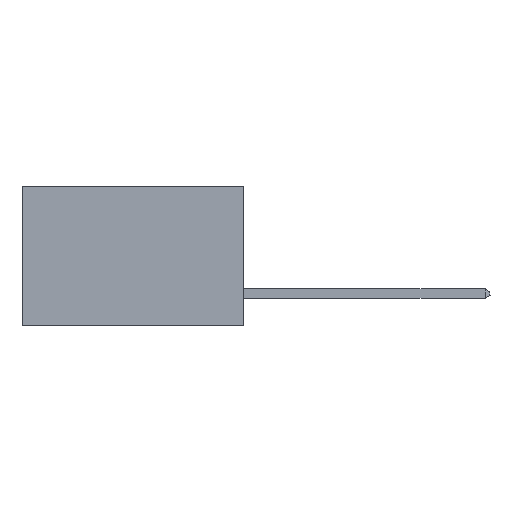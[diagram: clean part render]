
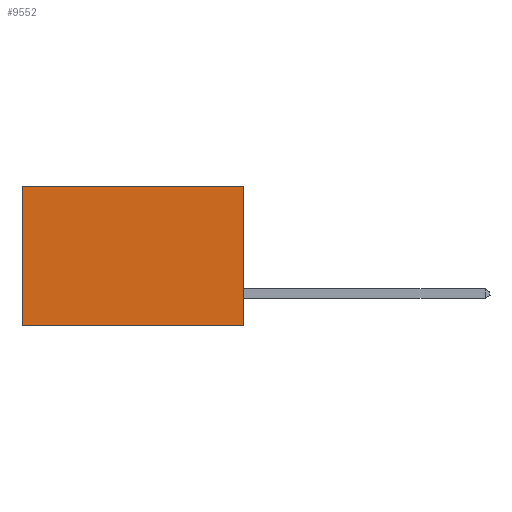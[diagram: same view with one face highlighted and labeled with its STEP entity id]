
A CAD part, left-side view. The second image highlights one B-rep face of the part: STEP entity #9552.
In plain terms, the highlighted planar face has unit normal (-1, 0, 0).
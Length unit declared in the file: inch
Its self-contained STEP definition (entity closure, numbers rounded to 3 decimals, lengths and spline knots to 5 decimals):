
#828 = CARTESIAN_POINT ( 'NONE',  ( 0.277, 0.59, 0. ) ) ;
#1208 = LINE ( 'NONE', #3026, #3178 ) ;
#1336 = EDGE_CURVE ( 'NONE', #2135, #3964, #9751, .T. ) ;
#1589 = LINE ( 'NONE', #7662, #7437 ) ;
#1812 = CARTESIAN_POINT ( 'NONE',  ( 0.277, 0., 0. ) ) ;
#2074 = VERTEX_POINT ( 'NONE', #828 ) ;
#2135 = VERTEX_POINT ( 'NONE', #4495 ) ;
#2694 = CARTESIAN_POINT ( 'NONE',  ( 0.277, 0., -0.37 ) ) ;
#3010 = DIRECTION ( 'NONE',  ( 0., 0., -1. ) ) ;
#3026 = CARTESIAN_POINT ( 'NONE',  ( 0.277, 0.59, -0.37 ) ) ;
#3117 = FACE_OUTER_BOUND ( 'NONE', #6435, .T. ) ;
#3178 = VECTOR ( 'NONE', #3010, 39.37008 ) ;
#3226 = EDGE_CURVE ( 'NONE', #4968, #2074, #1589, .T. ) ;
#3503 = VECTOR ( 'NONE', #6865, 39.37008 ) ;
#3539 = DIRECTION ( 'NONE',  ( 1., 0., 0. ) ) ;
#3964 = VERTEX_POINT ( 'NONE', #8629 ) ;
#4495 = CARTESIAN_POINT ( 'NONE',  ( 0.277, 0., -0.37 ) ) ;
#4794 = EDGE_CURVE ( 'NONE', #2074, #3964, #1208, .T. ) ;
#4968 = VERTEX_POINT ( 'NONE', #1812 ) ;
#5439 = DIRECTION ( 'NONE',  ( 0., 1., 0. ) ) ;
#5624 = ORIENTED_EDGE ( 'NONE', *, *, #1336, .F. ) ;
#5736 = AXIS2_PLACEMENT_3D ( 'NONE', #2694, #3539, #8880 ) ;
#5747 = CARTESIAN_POINT ( 'NONE',  ( 0.277, 0., -0.37 ) ) ;
#6435 = EDGE_LOOP ( 'NONE', ( #9334, #5624, #7628, #9555 ) ) ;
#6865 = DIRECTION ( 'NONE',  ( 0., 0., -1. ) ) ;
#7428 = PLANE ( 'NONE',  #5736 ) ;
#7437 = VECTOR ( 'NONE', #7481, 39.37008 ) ;
#7481 = DIRECTION ( 'NONE',  ( 0., 1., 0. ) ) ;
#7599 = VECTOR ( 'NONE', #5439, 39.37008 ) ;
#7628 = ORIENTED_EDGE ( 'NONE', *, *, #9847, .F. ) ;
#7639 = CARTESIAN_POINT ( 'NONE',  ( 0.277, 0., -0.37 ) ) ;
#7662 = CARTESIAN_POINT ( 'NONE',  ( 0.277, 0., 0. ) ) ;
#8629 = CARTESIAN_POINT ( 'NONE',  ( 0.277, 0.59, -0.37 ) ) ;
#8880 = DIRECTION ( 'NONE',  ( 0., 0., -1. ) ) ;
#9334 = ORIENTED_EDGE ( 'NONE', *, *, #4794, .T. ) ;
#9552 = ADVANCED_FACE ( 'NONE', ( #3117 ), #7428, .F. ) ;
#9555 = ORIENTED_EDGE ( 'NONE', *, *, #3226, .T. ) ;
#9565 = LINE ( 'NONE', #7639, #3503 ) ;
#9751 = LINE ( 'NONE', #5747, #7599 ) ;
#9847 = EDGE_CURVE ( 'NONE', #4968, #2135, #9565, .T. ) ;
